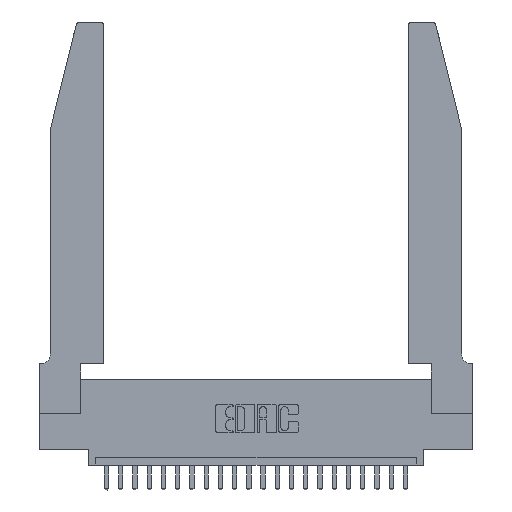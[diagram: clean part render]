
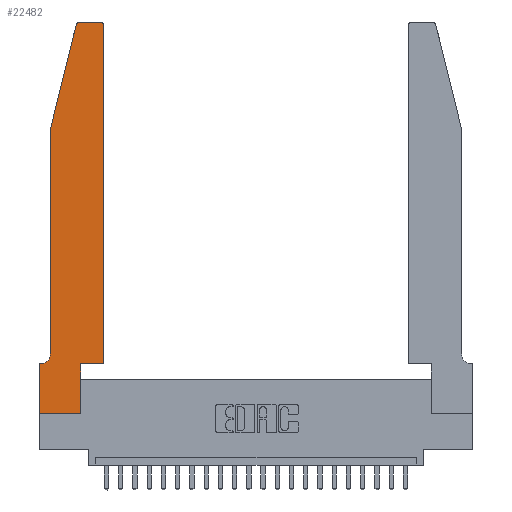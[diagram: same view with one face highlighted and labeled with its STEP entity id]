
A CAD part, top view. The second image highlights one B-rep face of the part: STEP entity #22482.
In plain terms, the highlighted planar face has unit normal (0, 0, 1).
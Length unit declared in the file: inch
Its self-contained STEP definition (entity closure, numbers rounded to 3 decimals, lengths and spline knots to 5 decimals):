
#63 = EDGE_CURVE ( 'NONE', #5103, #1280, #12880, .T. ) ;
#301 = VECTOR ( 'NONE', #22056, 39.37008 ) ;
#564 = DIRECTION ( 'NONE',  ( 1., 0., 0. ) ) ;
#803 = DIRECTION ( 'NONE',  ( -1., 0., 0. ) ) ;
#1280 = VERTEX_POINT ( 'NONE', #22732 ) ;
#1488 = VECTOR ( 'NONE', #16447, 39.37008 ) ;
#1533 = CARTESIAN_POINT ( 'NONE',  ( 0.4505, 0.35, 0.37 ) ) ;
#1567 = CARTESIAN_POINT ( 'NONE',  ( 0.284, 2.75, 0.37 ) ) ;
#1830 = VECTOR ( 'NONE', #22855, 39.37008 ) ;
#1976 = CARTESIAN_POINT ( 'NONE',  ( 0.4205, 2.75, 0.37 ) ) ;
#2003 = EDGE_CURVE ( 'NONE', #1280, #14881, #11894, .T. ) ;
#2043 = CARTESIAN_POINT ( 'NONE',  ( 0.2865, 0., 0.37 ) ) ;
#2068 = LINE ( 'NONE', #9226, #1488 ) ;
#2228 = EDGE_CURVE ( 'NONE', #3155, #7384, #22383, .T. ) ;
#2529 = CARTESIAN_POINT ( 'NONE',  ( 0.0055, 0.42, 0.37 ) ) ;
#2811 = EDGE_CURVE ( 'NONE', #6974, #14485, #15658, .T. ) ;
#3020 = VECTOR ( 'NONE', #10023, 39.37008 ) ;
#3155 = VERTEX_POINT ( 'NONE', #9905 ) ;
#3205 = DIRECTION ( 'NONE',  ( 1., 0., 0. ) ) ;
#3366 = CARTESIAN_POINT ( 'NONE',  ( 0.4205, 2.72, 0.37 ) ) ;
#3432 = EDGE_CURVE ( 'NONE', #21485, #19269, #20019, .T. ) ;
#3512 = AXIS2_PLACEMENT_3D ( 'NONE', #13534, #19155, #564 ) ;
#3719 = ORIENTED_EDGE ( 'NONE', *, *, #21437, .T. ) ;
#4216 = DIRECTION ( 'NONE',  ( 1., 0., 0. ) ) ;
#4658 = CARTESIAN_POINT ( 'NONE',  ( 0.0755, 2., 0.37 ) ) ;
#4752 = VECTOR ( 'NONE', #4216, 39.37008 ) ;
#5103 = VERTEX_POINT ( 'NONE', #1567 ) ;
#5142 = CARTESIAN_POINT ( 'NONE',  ( 0.0755, 2., 0.37 ) ) ;
#5393 = CARTESIAN_POINT ( 'NONE',  ( 0.2865, 0.35, 0.37 ) ) ;
#5635 = EDGE_CURVE ( 'NONE', #14881, #23991, #16771, .T. ) ;
#5667 = ORIENTED_EDGE ( 'NONE', *, *, #2228, .T. ) ;
#5735 = CARTESIAN_POINT ( 'NONE',  ( 0.4505, 0.35, 0.37 ) ) ;
#5737 = VERTEX_POINT ( 'NONE', #5393 ) ;
#6323 = VECTOR ( 'NONE', #7029, 39.37008 ) ;
#6414 = ORIENTED_EDGE ( 'NONE', *, *, #18657, .T. ) ;
#6974 = VERTEX_POINT ( 'NONE', #15817 ) ;
#7029 = DIRECTION ( 'NONE',  ( -0.239, -0.971, 0. ) ) ;
#7175 = CIRCLE ( 'NONE', #18295, 0.07 ) ;
#7384 = VERTEX_POINT ( 'NONE', #1976 ) ;
#7765 = ORIENTED_EDGE ( 'NONE', *, *, #24232, .T. ) ;
#8320 = VECTOR ( 'NONE', #23347, 39.37008 ) ;
#8463 = EDGE_CURVE ( 'NONE', #7384, #5103, #20387, .T. ) ;
#9120 = CARTESIAN_POINT ( 'NONE',  ( 0., 0.35, 0.37 ) ) ;
#9226 = CARTESIAN_POINT ( 'NONE',  ( 0.4505, 0.35, 0.37 ) ) ;
#9474 = CARTESIAN_POINT ( 'NONE',  ( 0., 0., 0.37 ) ) ;
#9713 = EDGE_CURVE ( 'NONE', #23991, #6974, #7175, .T. ) ;
#9742 = CARTESIAN_POINT ( 'NONE',  ( 0., 0., 0.37 ) ) ;
#9905 = CARTESIAN_POINT ( 'NONE',  ( 0.4505, 2.72, 0.37 ) ) ;
#9915 = ORIENTED_EDGE ( 'NONE', *, *, #3432, .T. ) ;
#10023 = DIRECTION ( 'NONE',  ( 0., 1., 0. ) ) ;
#10404 = VECTOR ( 'NONE', #21587, 39.37008 ) ;
#10530 = FACE_OUTER_BOUND ( 'NONE', #17900, .T. ) ;
#10767 = ORIENTED_EDGE ( 'NONE', *, *, #5635, .T. ) ;
#10815 = AXIS2_PLACEMENT_3D ( 'NONE', #16369, #18240, #12282 ) ;
#11894 = LINE ( 'NONE', #5142, #6323 ) ;
#12044 = CARTESIAN_POINT ( 'NONE',  ( 0.0755, 0.42, 0.37 ) ) ;
#12282 = DIRECTION ( 'NONE',  ( 1., 0., 0. ) ) ;
#12880 = CIRCLE ( 'NONE', #3512, 0.03 ) ;
#13485 = ORIENTED_EDGE ( 'NONE', *, *, #8463, .T. ) ;
#13534 = CARTESIAN_POINT ( 'NONE',  ( 0.284, 2.72, 0.37 ) ) ;
#13608 = LINE ( 'NONE', #19491, #3020 ) ;
#14001 = ORIENTED_EDGE ( 'NONE', *, *, #2811, .T. ) ;
#14255 = CARTESIAN_POINT ( 'NONE',  ( 0.0755, 0.35, 0.37 ) ) ;
#14485 = VERTEX_POINT ( 'NONE', #9120 ) ;
#14881 = VERTEX_POINT ( 'NONE', #4658 ) ;
#15142 = VERTEX_POINT ( 'NONE', #5735 ) ;
#15658 = LINE ( 'NONE', #14255, #10404 ) ;
#15817 = CARTESIAN_POINT ( 'NONE',  ( 0.0055, 0.35, 0.37 ) ) ;
#16369 = CARTESIAN_POINT ( 'NONE',  ( 0., 0.35, 0.37 ) ) ;
#16447 = DIRECTION ( 'NONE',  ( 0., 1., 0. ) ) ;
#16475 = LINE ( 'NONE', #1533, #301 ) ;
#16771 = LINE ( 'NONE', #17220, #1830 ) ;
#17139 = ORIENTED_EDGE ( 'NONE', *, *, #63, .T. ) ;
#17220 = CARTESIAN_POINT ( 'NONE',  ( 0.0755, 2., 0.37 ) ) ;
#17755 = DIRECTION ( 'NONE',  ( 0., 0., -1. ) ) ;
#17900 = EDGE_LOOP ( 'NONE', ( #13485, #17139, #18113, #10767, #23181, #14001, #6414, #9915, #20491, #7765, #3719, #5667 ) ) ;
#18113 = ORIENTED_EDGE ( 'NONE', *, *, #2003, .T. ) ;
#18240 = DIRECTION ( 'NONE',  ( 0., 0., 1. ) ) ;
#18295 = AXIS2_PLACEMENT_3D ( 'NONE', #2529, #17755, #803 ) ;
#18657 = EDGE_CURVE ( 'NONE', #14485, #21485, #22640, .T. ) ;
#19005 = EDGE_CURVE ( 'NONE', #19269, #5737, #13608, .T. ) ;
#19155 = DIRECTION ( 'NONE',  ( 0., 0., 1. ) ) ;
#19269 = VERTEX_POINT ( 'NONE', #2043 ) ;
#19491 = CARTESIAN_POINT ( 'NONE',  ( 0.2865, 0.35, 0.37 ) ) ;
#19673 = CARTESIAN_POINT ( 'NONE',  ( 0., 0., 0.37 ) ) ;
#20019 = LINE ( 'NONE', #9742, #4752 ) ;
#20077 = DIRECTION ( 'NONE',  ( -1., 0., 0. ) ) ;
#20080 = DIRECTION ( 'NONE',  ( 0., 0., 1. ) ) ;
#20387 = LINE ( 'NONE', #23162, #22731 ) ;
#20491 = ORIENTED_EDGE ( 'NONE', *, *, #19005, .T. ) ;
#21437 = EDGE_CURVE ( 'NONE', #15142, #3155, #2068, .T. ) ;
#21485 = VERTEX_POINT ( 'NONE', #9474 ) ;
#21587 = DIRECTION ( 'NONE',  ( -1., 0., 0. ) ) ;
#21812 = PLANE ( 'NONE',  #10815 ) ;
#22056 = DIRECTION ( 'NONE',  ( 1., 0., 0. ) ) ;
#22383 = CIRCLE ( 'NONE', #22820, 0.03 ) ;
#22482 = ADVANCED_FACE ( 'NONE', ( #10530 ), #21812, .T. ) ;
#22640 = LINE ( 'NONE', #19673, #8320 ) ;
#22731 = VECTOR ( 'NONE', #20077, 39.37008 ) ;
#22732 = CARTESIAN_POINT ( 'NONE',  ( 0.25487, 2.72718, 0.37 ) ) ;
#22820 = AXIS2_PLACEMENT_3D ( 'NONE', #3366, #20080, #3205 ) ;
#22855 = DIRECTION ( 'NONE',  ( 0., -1., 0. ) ) ;
#23162 = CARTESIAN_POINT ( 'NONE',  ( 0.2605, 2.75, 0.37 ) ) ;
#23181 = ORIENTED_EDGE ( 'NONE', *, *, #9713, .T. ) ;
#23347 = DIRECTION ( 'NONE',  ( 0., -1., 0. ) ) ;
#23991 = VERTEX_POINT ( 'NONE', #12044 ) ;
#24232 = EDGE_CURVE ( 'NONE', #5737, #15142, #16475, .T. ) ;
